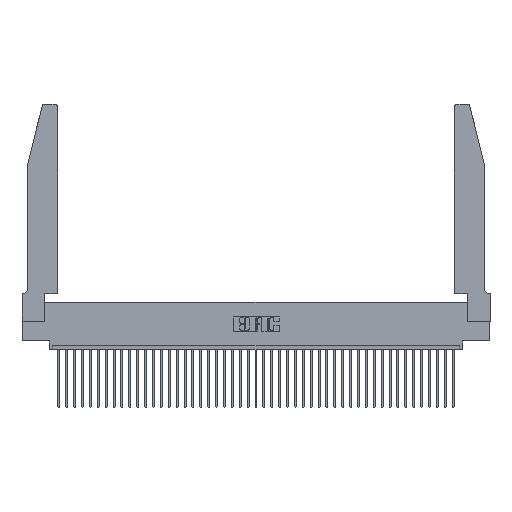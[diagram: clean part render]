
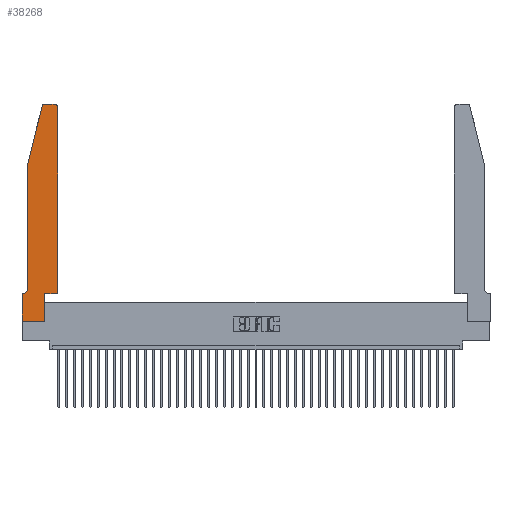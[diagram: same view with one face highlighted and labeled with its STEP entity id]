
A CAD part, top view. The second image highlights one B-rep face of the part: STEP entity #38268.
In plain terms, the highlighted planar face has unit normal (0, 0, 1).
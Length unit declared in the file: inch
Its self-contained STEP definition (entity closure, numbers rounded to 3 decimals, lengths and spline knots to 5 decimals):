
#421 = LINE ( 'NONE', #8563, #24822 ) ;
#701 = CARTESIAN_POINT ( 'NONE',  ( 0.284, 2.75, 0.37 ) ) ;
#717 = VERTEX_POINT ( 'NONE', #16661 ) ;
#936 = VERTEX_POINT ( 'NONE', #41653 ) ;
#1139 = ORIENTED_EDGE ( 'NONE', *, *, #39721, .T. ) ;
#1187 = DIRECTION ( 'NONE',  ( -1., 0., 0. ) ) ;
#1200 = DIRECTION ( 'NONE',  ( 0., 0., 1. ) ) ;
#1747 = ORIENTED_EDGE ( 'NONE', *, *, #33777, .T. ) ;
#1769 = AXIS2_PLACEMENT_3D ( 'NONE', #35327, #3107, #15684 ) ;
#2090 = CIRCLE ( 'NONE', #7772, 0.03 ) ;
#2776 = CARTESIAN_POINT ( 'NONE',  ( 0.0755, 2., 0.37 ) ) ;
#2888 = VERTEX_POINT ( 'NONE', #14596 ) ;
#3107 = DIRECTION ( 'NONE',  ( 0., 0., 1. ) ) ;
#3399 = VECTOR ( 'NONE', #21815, 39.37008 ) ;
#4466 = LINE ( 'NONE', #27120, #34938 ) ;
#4565 = LINE ( 'NONE', #36131, #20787 ) ;
#4743 = VERTEX_POINT ( 'NONE', #7384 ) ;
#5386 = DIRECTION ( 'NONE',  ( -1., 0., 0. ) ) ;
#5498 = VERTEX_POINT ( 'NONE', #22725 ) ;
#6222 = CARTESIAN_POINT ( 'NONE',  ( 0.0055, 0.35, 0.37 ) ) ;
#6236 = CARTESIAN_POINT ( 'NONE',  ( 0.0755, 0.42, 0.37 ) ) ;
#7022 = LINE ( 'NONE', #12174, #31904 ) ;
#7150 = AXIS2_PLACEMENT_3D ( 'NONE', #27019, #1200, #40365 ) ;
#7269 = DIRECTION ( 'NONE',  ( -1., 0., 0. ) ) ;
#7384 = CARTESIAN_POINT ( 'NONE',  ( 0.25487, 2.72718, 0.37 ) ) ;
#7468 = CARTESIAN_POINT ( 'NONE',  ( 0.4205, 2.72, 0.37 ) ) ;
#7720 = CARTESIAN_POINT ( 'NONE',  ( 0.0055, 0.42, 0.37 ) ) ;
#7772 = AXIS2_PLACEMENT_3D ( 'NONE', #7468, #10736, #33453 ) ;
#8563 = CARTESIAN_POINT ( 'NONE',  ( 0., 0., 0.37 ) ) ;
#8817 = DIRECTION ( 'NONE',  ( 1., 0., 0. ) ) ;
#9128 = VECTOR ( 'NONE', #11950, 39.37008 ) ;
#10607 = EDGE_CURVE ( 'NONE', #13881, #12339, #33056, .T. ) ;
#10736 = DIRECTION ( 'NONE',  ( 0., 0., 1. ) ) ;
#11950 = DIRECTION ( 'NONE',  ( 1., 0., 0. ) ) ;
#12174 = CARTESIAN_POINT ( 'NONE',  ( 0.2605, 2.75, 0.37 ) ) ;
#12339 = VERTEX_POINT ( 'NONE', #6236 ) ;
#12366 = CARTESIAN_POINT ( 'NONE',  ( 0., 0.35, 0.37 ) ) ;
#12834 = EDGE_CURVE ( 'NONE', #36074, #717, #37447, .T. ) ;
#13420 = EDGE_CURVE ( 'NONE', #12339, #32096, #28217, .T. ) ;
#13881 = VERTEX_POINT ( 'NONE', #2776 ) ;
#14596 = CARTESIAN_POINT ( 'NONE',  ( 0.4205, 2.75, 0.37 ) ) ;
#15552 = CARTESIAN_POINT ( 'NONE',  ( 0., 0., 0.37 ) ) ;
#15655 = CARTESIAN_POINT ( 'NONE',  ( 0.4505, 0.35, 0.37 ) ) ;
#15684 = DIRECTION ( 'NONE',  ( 1., 0., 0. ) ) ;
#16661 = CARTESIAN_POINT ( 'NONE',  ( 0.4505, 2.72, 0.37 ) ) ;
#16690 = EDGE_CURVE ( 'NONE', #936, #36074, #24349, .T. ) ;
#17630 = PLANE ( 'NONE',  #7150 ) ;
#18308 = VECTOR ( 'NONE', #8817, 39.37008 ) ;
#18792 = ORIENTED_EDGE ( 'NONE', *, *, #12834, .T. ) ;
#19268 = DIRECTION ( 'NONE',  ( -0.239, -0.971, 0. ) ) ;
#19350 = LINE ( 'NONE', #15552, #18308 ) ;
#19426 = ORIENTED_EDGE ( 'NONE', *, *, #16690, .T. ) ;
#19881 = VERTEX_POINT ( 'NONE', #12366 ) ;
#20787 = VECTOR ( 'NONE', #29176, 39.37008 ) ;
#20830 = AXIS2_PLACEMENT_3D ( 'NONE', #7720, #30719, #1187 ) ;
#21455 = EDGE_CURVE ( 'NONE', #717, #2888, #2090, .T. ) ;
#21815 = DIRECTION ( 'NONE',  ( 0., 1., 0. ) ) ;
#21993 = EDGE_CURVE ( 'NONE', #5498, #936, #4565, .T. ) ;
#22296 = EDGE_LOOP ( 'NONE', ( #1747, #1139, #36000, #24204, #28083, #32644, #22792, #34489, #35179, #19426, #18792, #39379 ) ) ;
#22358 = EDGE_CURVE ( 'NONE', #19881, #24158, #421, .T. ) ;
#22725 = CARTESIAN_POINT ( 'NONE',  ( 0.2865, 0., 0.37 ) ) ;
#22792 = ORIENTED_EDGE ( 'NONE', *, *, #22358, .T. ) ;
#23251 = VERTEX_POINT ( 'NONE', #701 ) ;
#24158 = VERTEX_POINT ( 'NONE', #39006 ) ;
#24204 = ORIENTED_EDGE ( 'NONE', *, *, #10607, .T. ) ;
#24349 = LINE ( 'NONE', #31403, #9128 ) ;
#24822 = VECTOR ( 'NONE', #35100, 39.37008 ) ;
#26742 = EDGE_CURVE ( 'NONE', #24158, #5498, #19350, .T. ) ;
#27019 = CARTESIAN_POINT ( 'NONE',  ( 0., 0.35, 0.37 ) ) ;
#27120 = CARTESIAN_POINT ( 'NONE',  ( 0.0755, 0.35, 0.37 ) ) ;
#28083 = ORIENTED_EDGE ( 'NONE', *, *, #13420, .T. ) ;
#28217 = CIRCLE ( 'NONE', #20830, 0.07 ) ;
#28571 = EDGE_CURVE ( 'NONE', #32096, #19881, #4466, .T. ) ;
#29176 = DIRECTION ( 'NONE',  ( 0., 1., 0. ) ) ;
#29212 = CARTESIAN_POINT ( 'NONE',  ( 0.0755, 2., 0.37 ) ) ;
#30719 = DIRECTION ( 'NONE',  ( 0., 0., -1. ) ) ;
#30873 = CIRCLE ( 'NONE', #1769, 0.03 ) ;
#30990 = DIRECTION ( 'NONE',  ( 0., -1., 0. ) ) ;
#31403 = CARTESIAN_POINT ( 'NONE',  ( 0.4505, 0.35, 0.37 ) ) ;
#31904 = VECTOR ( 'NONE', #5386, 39.37008 ) ;
#32096 = VERTEX_POINT ( 'NONE', #6222 ) ;
#32644 = ORIENTED_EDGE ( 'NONE', *, *, #28571, .T. ) ;
#33056 = LINE ( 'NONE', #40630, #33541 ) ;
#33453 = DIRECTION ( 'NONE',  ( 1., 0., 0. ) ) ;
#33536 = FACE_OUTER_BOUND ( 'NONE', #22296, .T. ) ;
#33541 = VECTOR ( 'NONE', #30990, 39.37008 ) ;
#33777 = EDGE_CURVE ( 'NONE', #2888, #23251, #7022, .T. ) ;
#34489 = ORIENTED_EDGE ( 'NONE', *, *, #26742, .T. ) ;
#34938 = VECTOR ( 'NONE', #7269, 39.37008 ) ;
#35100 = DIRECTION ( 'NONE',  ( 0., -1., 0. ) ) ;
#35179 = ORIENTED_EDGE ( 'NONE', *, *, #21993, .T. ) ;
#35327 = CARTESIAN_POINT ( 'NONE',  ( 0.284, 2.72, 0.37 ) ) ;
#36000 = ORIENTED_EDGE ( 'NONE', *, *, #39664, .T. ) ;
#36074 = VERTEX_POINT ( 'NONE', #37960 ) ;
#36131 = CARTESIAN_POINT ( 'NONE',  ( 0.2865, 0.35, 0.37 ) ) ;
#37447 = LINE ( 'NONE', #15655, #3399 ) ;
#37960 = CARTESIAN_POINT ( 'NONE',  ( 0.4505, 0.35, 0.37 ) ) ;
#38268 = ADVANCED_FACE ( 'NONE', ( #33536 ), #17630, .T. ) ;
#39006 = CARTESIAN_POINT ( 'NONE',  ( 0., 0., 0.37 ) ) ;
#39379 = ORIENTED_EDGE ( 'NONE', *, *, #21455, .T. ) ;
#39664 = EDGE_CURVE ( 'NONE', #4743, #13881, #41573, .T. ) ;
#39721 = EDGE_CURVE ( 'NONE', #23251, #4743, #30873, .T. ) ;
#40014 = VECTOR ( 'NONE', #19268, 39.37008 ) ;
#40365 = DIRECTION ( 'NONE',  ( 1., 0., 0. ) ) ;
#40630 = CARTESIAN_POINT ( 'NONE',  ( 0.0755, 2., 0.37 ) ) ;
#41573 = LINE ( 'NONE', #29212, #40014 ) ;
#41653 = CARTESIAN_POINT ( 'NONE',  ( 0.2865, 0.35, 0.37 ) ) ;
